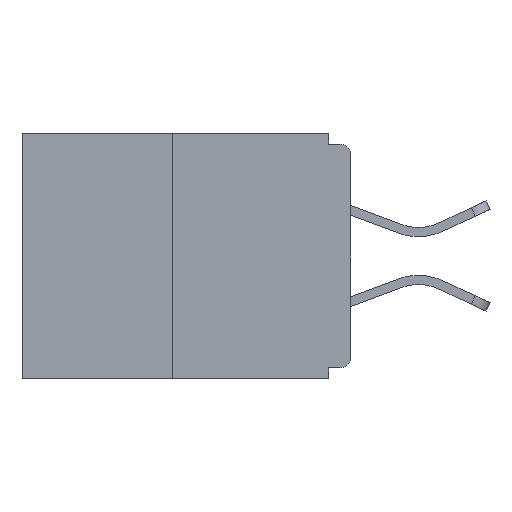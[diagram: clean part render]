
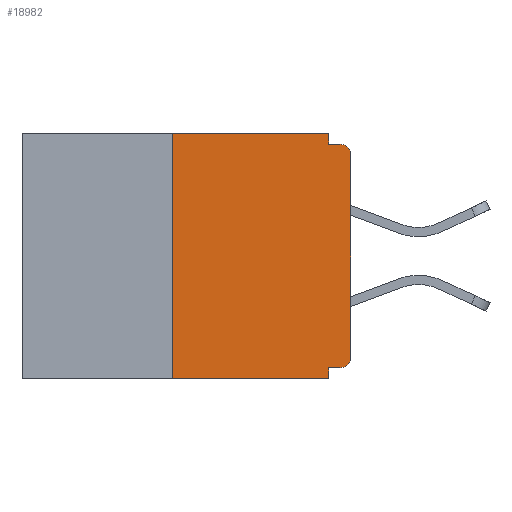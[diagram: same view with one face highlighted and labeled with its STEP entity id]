
A CAD part, left-side view. The second image highlights one B-rep face of the part: STEP entity #18982.
In plain terms, the highlighted planar face has unit normal (-1, 0, 0).
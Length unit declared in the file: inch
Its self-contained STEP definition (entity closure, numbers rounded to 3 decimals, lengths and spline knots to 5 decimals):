
#318 = EDGE_LOOP ( 'NONE', ( #21054, #25760, #3802, #9255, #1579, #2004, #1792, #4240, #30904, #20231 ) ) ;
#488 = EDGE_CURVE ( 'NONE', #2817, #8262, #1891, .T. ) ;
#943 = LINE ( 'NONE', #30240, #13449 ) ;
#1244 = VECTOR ( 'NONE', #6499, 39.37008 ) ;
#1283 = VERTEX_POINT ( 'NONE', #7561 ) ;
#1524 = CARTESIAN_POINT ( 'NONE',  ( 0., 0.031, -0.328 ) ) ;
#1579 = ORIENTED_EDGE ( 'NONE', *, *, #26606, .F. ) ;
#1792 = ORIENTED_EDGE ( 'NONE', *, *, #488, .T. ) ;
#1891 = LINE ( 'NONE', #20372, #12851 ) ;
#2000 = DIRECTION ( 'NONE',  ( 0., 1., 0. ) ) ;
#2004 = ORIENTED_EDGE ( 'NONE', *, *, #24478, .T. ) ;
#2018 = EDGE_CURVE ( 'NONE', #29544, #8323, #25717, .T. ) ;
#2789 = CARTESIAN_POINT ( 'NONE',  ( 0., 0.031, -0.343 ) ) ;
#2817 = VERTEX_POINT ( 'NONE', #22233 ) ;
#2937 = LINE ( 'NONE', #14377, #19781 ) ;
#2959 = VECTOR ( 'NONE', #3153, 39.37008 ) ;
#3081 = EDGE_CURVE ( 'NONE', #15373, #29544, #16269, .T. ) ;
#3153 = DIRECTION ( 'NONE',  ( 0., -1., 0. ) ) ;
#3802 = ORIENTED_EDGE ( 'NONE', *, *, #16158, .T. ) ;
#4240 = ORIENTED_EDGE ( 'NONE', *, *, #24604, .T. ) ;
#6499 = DIRECTION ( 'NONE',  ( 0., 0., 1. ) ) ;
#6679 = AXIS2_PLACEMENT_3D ( 'NONE', #12675, #12790, #17384 ) ;
#7229 = CIRCLE ( 'NONE', #21927, 0.015 ) ;
#7378 = DIRECTION ( 'NONE',  ( 0., -1., 0. ) ) ;
#7561 = CARTESIAN_POINT ( 'NONE',  ( 0., 0.25, -0.343 ) ) ;
#8262 = VERTEX_POINT ( 'NONE', #11398 ) ;
#8323 = VERTEX_POINT ( 'NONE', #14116 ) ;
#9255 = ORIENTED_EDGE ( 'NONE', *, *, #27616, .F. ) ;
#9307 = DIRECTION ( 'NONE',  ( 0., -1., 0. ) ) ;
#9370 = VECTOR ( 'NONE', #9307, 39.37008 ) ;
#9910 = LINE ( 'NONE', #2789, #22423 ) ;
#10203 = VERTEX_POINT ( 'NONE', #1524 ) ;
#10271 = CARTESIAN_POINT ( 'NONE',  ( 0., 0.031, -0.343 ) ) ;
#11009 = CARTESIAN_POINT ( 'NONE',  ( 0., 0.25, 0. ) ) ;
#11398 = CARTESIAN_POINT ( 'NONE',  ( 0., 0., -0.03 ) ) ;
#12164 = CARTESIAN_POINT ( 'NONE',  ( 0., 0.015, -0.328 ) ) ;
#12509 = FACE_OUTER_BOUND ( 'NONE', #318, .T. ) ;
#12675 = CARTESIAN_POINT ( 'NONE',  ( 0., 0.46, 0. ) ) ;
#12790 = DIRECTION ( 'NONE',  ( 1., 0., 0. ) ) ;
#12812 = CARTESIAN_POINT ( 'NONE',  ( 0., 0.46, 0. ) ) ;
#12851 = VECTOR ( 'NONE', #25421, 39.37008 ) ;
#13335 = CARTESIAN_POINT ( 'NONE',  ( 0., 0.015, -0.313 ) ) ;
#13449 = VECTOR ( 'NONE', #7378, 39.37008 ) ;
#14116 = CARTESIAN_POINT ( 'NONE',  ( 0., 0.031, -0.015 ) ) ;
#14228 = CARTESIAN_POINT ( 'NONE',  ( 0., 0.46, -0.343 ) ) ;
#14377 = CARTESIAN_POINT ( 'NONE',  ( 0., 0., -0.328 ) ) ;
#15002 = CARTESIAN_POINT ( 'NONE',  ( 0., 0.031, 0. ) ) ;
#15373 = VERTEX_POINT ( 'NONE', #11009 ) ;
#16055 = DIRECTION ( 'NONE',  ( -1., 0., 0. ) ) ;
#16158 = EDGE_CURVE ( 'NONE', #1283, #18974, #28642, .T. ) ;
#16269 = LINE ( 'NONE', #12812, #2959 ) ;
#17033 = DIRECTION ( 'NONE',  ( 0., 0., -1. ) ) ;
#17384 = DIRECTION ( 'NONE',  ( 0., 0., -1. ) ) ;
#17897 = DIRECTION ( 'NONE',  ( 0., 0., -1. ) ) ;
#18607 = DIRECTION ( 'NONE',  ( 0., 0., -1. ) ) ;
#18974 = VERTEX_POINT ( 'NONE', #10271 ) ;
#18982 = ADVANCED_FACE ( 'NONE', ( #12509 ), #22512, .F. ) ;
#19046 = VECTOR ( 'NONE', #17033, 39.37008 ) ;
#19759 = VERTEX_POINT ( 'NONE', #31749 ) ;
#19781 = VECTOR ( 'NONE', #2000, 39.37008 ) ;
#20231 = ORIENTED_EDGE ( 'NONE', *, *, #2018, .F. ) ;
#20372 = CARTESIAN_POINT ( 'NONE',  ( 0., 0., 0. ) ) ;
#21054 = ORIENTED_EDGE ( 'NONE', *, *, #3081, .F. ) ;
#21227 = LINE ( 'NONE', #26316, #1244 ) ;
#21927 = AXIS2_PLACEMENT_3D ( 'NONE', #31084, #16055, #18607 ) ;
#22080 = CIRCLE ( 'NONE', #30779, 0.015 ) ;
#22233 = CARTESIAN_POINT ( 'NONE',  ( 0., 0., -0.313 ) ) ;
#22423 = VECTOR ( 'NONE', #17897, 39.37008 ) ;
#22512 = PLANE ( 'NONE',  #6679 ) ;
#24025 = CARTESIAN_POINT ( 'NONE',  ( 0., 0.031, 0. ) ) ;
#24478 = EDGE_CURVE ( 'NONE', #29757, #2817, #22080, .T. ) ;
#24604 = EDGE_CURVE ( 'NONE', #8262, #19759, #7229, .T. ) ;
#25421 = DIRECTION ( 'NONE',  ( 0., 0., 1. ) ) ;
#25717 = LINE ( 'NONE', #24025, #19046 ) ;
#25760 = ORIENTED_EDGE ( 'NONE', *, *, #32039, .F. ) ;
#26316 = CARTESIAN_POINT ( 'NONE',  ( 0., 0.25, 0. ) ) ;
#26606 = EDGE_CURVE ( 'NONE', #29757, #10203, #2937, .T. ) ;
#27616 = EDGE_CURVE ( 'NONE', #10203, #18974, #9910, .T. ) ;
#28469 = DIRECTION ( 'NONE',  ( -1., 0., 0. ) ) ;
#28642 = LINE ( 'NONE', #14228, #9370 ) ;
#28787 = DIRECTION ( 'NONE',  ( 0., 0., -1. ) ) ;
#29544 = VERTEX_POINT ( 'NONE', #15002 ) ;
#29757 = VERTEX_POINT ( 'NONE', #12164 ) ;
#30240 = CARTESIAN_POINT ( 'NONE',  ( 0., 0., -0.015 ) ) ;
#30421 = EDGE_CURVE ( 'NONE', #8323, #19759, #943, .T. ) ;
#30779 = AXIS2_PLACEMENT_3D ( 'NONE', #13335, #28469, #28787 ) ;
#30904 = ORIENTED_EDGE ( 'NONE', *, *, #30421, .F. ) ;
#31084 = CARTESIAN_POINT ( 'NONE',  ( 0., 0.015, -0.03 ) ) ;
#31749 = CARTESIAN_POINT ( 'NONE',  ( 0., 0.015, -0.015 ) ) ;
#32039 = EDGE_CURVE ( 'NONE', #1283, #15373, #21227, .T. ) ;
